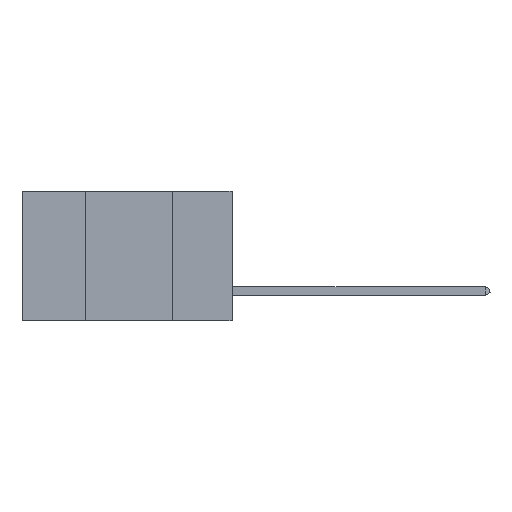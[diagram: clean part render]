
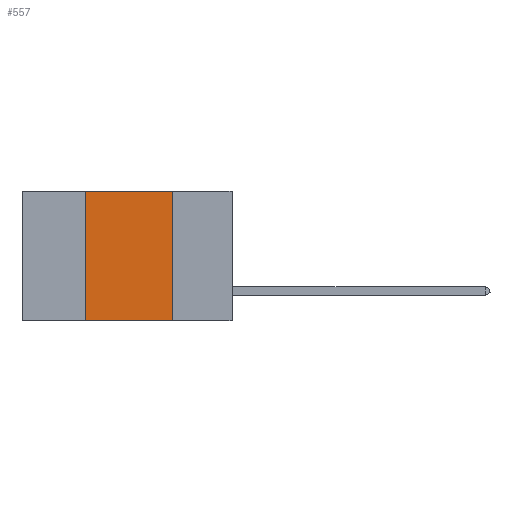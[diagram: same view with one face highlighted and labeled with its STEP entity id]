
A CAD part, left-side view. The second image highlights one B-rep face of the part: STEP entity #557.
In plain terms, the highlighted planar face has unit normal (-1, 0, 0).
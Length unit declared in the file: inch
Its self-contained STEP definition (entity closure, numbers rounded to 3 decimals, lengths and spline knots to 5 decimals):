
#234 = LINE ( 'NONE', #3481, #20594 ) ;
#557 = ADVANCED_FACE ( 'NONE', ( #9350 ), #6676, .F. ) ;
#2866 = VERTEX_POINT ( 'NONE', #14100 ) ;
#3481 = CARTESIAN_POINT ( 'NONE',  ( 0., 0.6, -0.37 ) ) ;
#3659 = CARTESIAN_POINT ( 'NONE',  ( 0., 0.6, 0. ) ) ;
#5511 = CARTESIAN_POINT ( 'NONE',  ( 0., 0.17, 0. ) ) ;
#5681 = DIRECTION ( 'NONE',  ( 1., 0., 0. ) ) ;
#6676 = PLANE ( 'NONE',  #15145 ) ;
#6776 = ORIENTED_EDGE ( 'NONE', *, *, #17923, .T. ) ;
#7563 = CARTESIAN_POINT ( 'NONE',  ( 0., 0.17, 0. ) ) ;
#8014 = LINE ( 'NONE', #7563, #11049 ) ;
#9148 = ORIENTED_EDGE ( 'NONE', *, *, #20987, .F. ) ;
#9350 = FACE_OUTER_BOUND ( 'NONE', #9396, .T. ) ;
#9396 = EDGE_LOOP ( 'NONE', ( #11707, #13405, #9148, #6776 ) ) ;
#9500 = VERTEX_POINT ( 'NONE', #16525 ) ;
#9946 = DIRECTION ( 'NONE',  ( 0., 0., -1. ) ) ;
#10650 = CARTESIAN_POINT ( 'NONE',  ( 0., 0.17, -0.37 ) ) ;
#11049 = VECTOR ( 'NONE', #9946, 39.37008 ) ;
#11145 = EDGE_CURVE ( 'NONE', #9500, #18190, #14528, .T. ) ;
#11707 = ORIENTED_EDGE ( 'NONE', *, *, #19960, .F. ) ;
#11915 = VERTEX_POINT ( 'NONE', #10650 ) ;
#12669 = CARTESIAN_POINT ( 'NONE',  ( 0., 0.42, 0. ) ) ;
#12689 = LINE ( 'NONE', #12669, #17534 ) ;
#13125 = DIRECTION ( 'NONE',  ( 0., -1., 0. ) ) ;
#13405 = ORIENTED_EDGE ( 'NONE', *, *, #11145, .F. ) ;
#14100 = CARTESIAN_POINT ( 'NONE',  ( 0., 0.42, -0.37 ) ) ;
#14528 = LINE ( 'NONE', #3659, #17836 ) ;
#15010 = DIRECTION ( 'NONE',  ( 0., -1., 0. ) ) ;
#15145 = AXIS2_PLACEMENT_3D ( 'NONE', #15420, #5681, #20695 ) ;
#15420 = CARTESIAN_POINT ( 'NONE',  ( 0., 0.6, 0. ) ) ;
#16525 = CARTESIAN_POINT ( 'NONE',  ( 0., 0.42, 0. ) ) ;
#17534 = VECTOR ( 'NONE', #20901, 39.37008 ) ;
#17836 = VECTOR ( 'NONE', #15010, 39.37008 ) ;
#17923 = EDGE_CURVE ( 'NONE', #2866, #11915, #234, .T. ) ;
#18190 = VERTEX_POINT ( 'NONE', #5511 ) ;
#19960 = EDGE_CURVE ( 'NONE', #18190, #11915, #8014, .T. ) ;
#20594 = VECTOR ( 'NONE', #13125, 39.37008 ) ;
#20695 = DIRECTION ( 'NONE',  ( 0., 0., -1. ) ) ;
#20901 = DIRECTION ( 'NONE',  ( 0., 0., 1. ) ) ;
#20987 = EDGE_CURVE ( 'NONE', #2866, #9500, #12689, .T. ) ;
